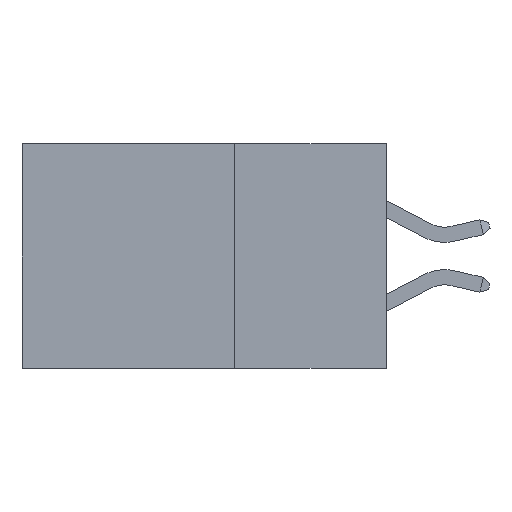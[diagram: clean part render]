
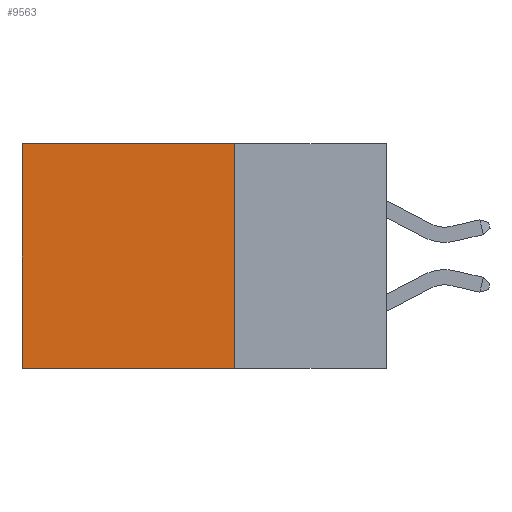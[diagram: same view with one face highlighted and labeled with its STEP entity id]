
A CAD part, left-side view. The second image highlights one B-rep face of the part: STEP entity #9563.
In plain terms, the highlighted planar face has unit normal (-1, 0, 0).
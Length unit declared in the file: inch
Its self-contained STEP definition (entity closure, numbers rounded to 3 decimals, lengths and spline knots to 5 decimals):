
#838 = CARTESIAN_POINT ( 'NONE',  ( 0.2615, 0.6, -0.37 ) ) ;
#4122 = VERTEX_POINT ( 'NONE', #18408 ) ;
#4597 = CARTESIAN_POINT ( 'NONE',  ( 0.2615, 0.25, 0. ) ) ;
#4980 = ORIENTED_EDGE ( 'NONE', *, *, #25062, .F. ) ;
#5091 = CARTESIAN_POINT ( 'NONE',  ( 0.2615, 0.6, -0.37 ) ) ;
#5274 = LINE ( 'NONE', #838, #20807 ) ;
#5337 = VERTEX_POINT ( 'NONE', #5091 ) ;
#5377 = EDGE_CURVE ( 'NONE', #13781, #5337, #22321, .T. ) ;
#5440 = ORIENTED_EDGE ( 'NONE', *, *, #6639, .T. ) ;
#6639 = EDGE_CURVE ( 'NONE', #27246, #5337, #5274, .T. ) ;
#7593 = DIRECTION ( 'NONE',  ( 0., 1., 0. ) ) ;
#9325 = DIRECTION ( 'NONE',  ( 0., 0., -1. ) ) ;
#9520 = PLANE ( 'NONE',  #22589 ) ;
#9563 = ADVANCED_FACE ( 'NONE', ( #11607 ), #9520, .F. ) ;
#10441 = CARTESIAN_POINT ( 'NONE',  ( 0.2615, 0.25, -0.37 ) ) ;
#11413 = VECTOR ( 'NONE', #16538, 39.37008 ) ;
#11607 = FACE_OUTER_BOUND ( 'NONE', #19081, .T. ) ;
#12190 = ORIENTED_EDGE ( 'NONE', *, *, #20926, .T. ) ;
#13781 = VERTEX_POINT ( 'NONE', #27020 ) ;
#13853 = CARTESIAN_POINT ( 'NONE',  ( 0.2615, 0.6, 0. ) ) ;
#15309 = DIRECTION ( 'NONE',  ( 0., 1., 0. ) ) ;
#15440 = LINE ( 'NONE', #4597, #27239 ) ;
#15865 = VECTOR ( 'NONE', #7593, 39.37008 ) ;
#16249 = ORIENTED_EDGE ( 'NONE', *, *, #5377, .F. ) ;
#16538 = DIRECTION ( 'NONE',  ( 0., 0., -1. ) ) ;
#17982 = CARTESIAN_POINT ( 'NONE',  ( 0.2615, 0.25, -0.37 ) ) ;
#18243 = DIRECTION ( 'NONE',  ( 1., 0., 0. ) ) ;
#18408 = CARTESIAN_POINT ( 'NONE',  ( 0.2615, 0.25, 0. ) ) ;
#19081 = EDGE_LOOP ( 'NONE', ( #5440, #16249, #4980, #12190 ) ) ;
#20807 = VECTOR ( 'NONE', #9325, 39.37008 ) ;
#20926 = EDGE_CURVE ( 'NONE', #4122, #27246, #15440, .T. ) ;
#22321 = LINE ( 'NONE', #26615, #15865 ) ;
#22589 = AXIS2_PLACEMENT_3D ( 'NONE', #17982, #18243, #26715 ) ;
#25062 = EDGE_CURVE ( 'NONE', #4122, #13781, #25293, .T. ) ;
#25293 = LINE ( 'NONE', #10441, #11413 ) ;
#26615 = CARTESIAN_POINT ( 'NONE',  ( 0.2615, 0.25, -0.37 ) ) ;
#26715 = DIRECTION ( 'NONE',  ( 0., 0., -1. ) ) ;
#27020 = CARTESIAN_POINT ( 'NONE',  ( 0.2615, 0.25, -0.37 ) ) ;
#27239 = VECTOR ( 'NONE', #15309, 39.37008 ) ;
#27246 = VERTEX_POINT ( 'NONE', #13853 ) ;
